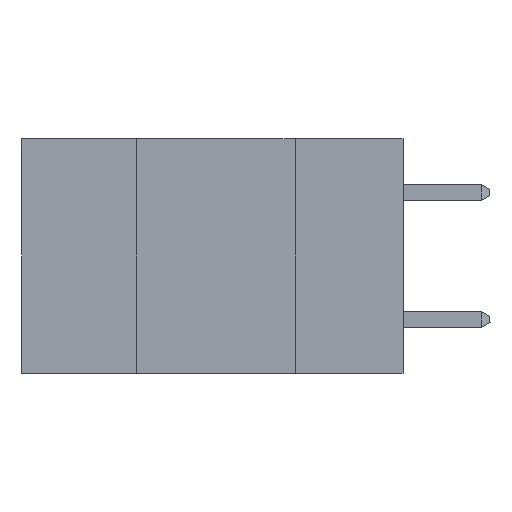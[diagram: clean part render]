
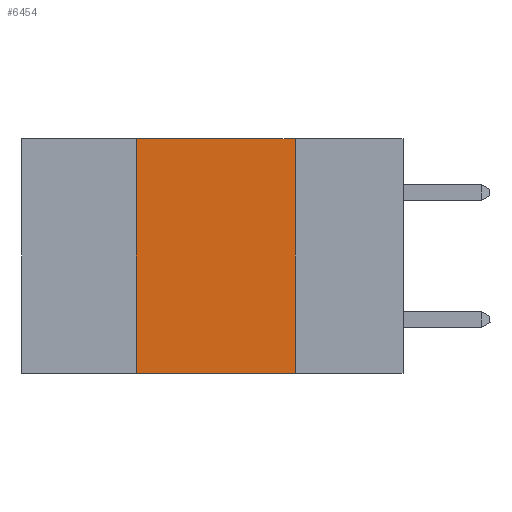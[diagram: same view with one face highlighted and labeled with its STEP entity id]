
A CAD part, left-side view. The second image highlights one B-rep face of the part: STEP entity #6454.
In plain terms, the highlighted planar face has unit normal (-1, 0, 0).
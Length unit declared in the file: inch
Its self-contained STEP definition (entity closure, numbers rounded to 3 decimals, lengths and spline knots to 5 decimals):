
#899 = CARTESIAN_POINT ( 'NONE',  ( 0., 0.6, -0.37 ) ) ;
#2065 = FACE_OUTER_BOUND ( 'NONE', #6044, .T. ) ;
#3694 = ORIENTED_EDGE ( 'NONE', *, *, #24205, .F. ) ;
#3903 = VERTEX_POINT ( 'NONE', #15027 ) ;
#3914 = CARTESIAN_POINT ( 'NONE',  ( 0., 0.42, 0. ) ) ;
#4265 = LINE ( 'NONE', #8884, #32738 ) ;
#5208 = DIRECTION ( 'NONE',  ( 0., 0., -1. ) ) ;
#6044 = EDGE_LOOP ( 'NONE', ( #11949, #3694, #11099, #32468 ) ) ;
#6332 = CARTESIAN_POINT ( 'NONE',  ( 0., 0.17, -0.37 ) ) ;
#6454 = ADVANCED_FACE ( 'NONE', ( #2065 ), #30479, .F. ) ;
#8111 = LINE ( 'NONE', #25490, #32905 ) ;
#8884 = CARTESIAN_POINT ( 'NONE',  ( 0., 0.17, 0. ) ) ;
#9180 = DIRECTION ( 'NONE',  ( 0., 0., 1. ) ) ;
#9628 = EDGE_CURVE ( 'NONE', #3903, #14246, #4265, .T. ) ;
#9678 = AXIS2_PLACEMENT_3D ( 'NONE', #25274, #17466, #22729 ) ;
#11099 = ORIENTED_EDGE ( 'NONE', *, *, #20150, .F. ) ;
#11554 = VECTOR ( 'NONE', #19308, 39.37008 ) ;
#11577 = EDGE_CURVE ( 'NONE', #22549, #14246, #14415, .T. ) ;
#11949 = ORIENTED_EDGE ( 'NONE', *, *, #9628, .F. ) ;
#12346 = CARTESIAN_POINT ( 'NONE',  ( 0., 0.42, 0. ) ) ;
#13591 = CARTESIAN_POINT ( 'NONE',  ( 0., 0.42, -0.37 ) ) ;
#14246 = VERTEX_POINT ( 'NONE', #6332 ) ;
#14415 = LINE ( 'NONE', #899, #11554 ) ;
#15027 = CARTESIAN_POINT ( 'NONE',  ( 0., 0.17, 0. ) ) ;
#17466 = DIRECTION ( 'NONE',  ( 1., 0., 0. ) ) ;
#17938 = VERTEX_POINT ( 'NONE', #12346 ) ;
#19308 = DIRECTION ( 'NONE',  ( 0., -1., 0. ) ) ;
#20150 = EDGE_CURVE ( 'NONE', #22549, #17938, #32794, .T. ) ;
#20328 = DIRECTION ( 'NONE',  ( 0., -1., 0. ) ) ;
#22549 = VERTEX_POINT ( 'NONE', #13591 ) ;
#22729 = DIRECTION ( 'NONE',  ( 0., 0., -1. ) ) ;
#24205 = EDGE_CURVE ( 'NONE', #17938, #3903, #8111, .T. ) ;
#25274 = CARTESIAN_POINT ( 'NONE',  ( 0., 0.6, 0. ) ) ;
#25490 = CARTESIAN_POINT ( 'NONE',  ( 0., 0.6, 0. ) ) ;
#30395 = VECTOR ( 'NONE', #9180, 39.37008 ) ;
#30479 = PLANE ( 'NONE',  #9678 ) ;
#32468 = ORIENTED_EDGE ( 'NONE', *, *, #11577, .T. ) ;
#32738 = VECTOR ( 'NONE', #5208, 39.37008 ) ;
#32794 = LINE ( 'NONE', #3914, #30395 ) ;
#32905 = VECTOR ( 'NONE', #20328, 39.37008 ) ;
